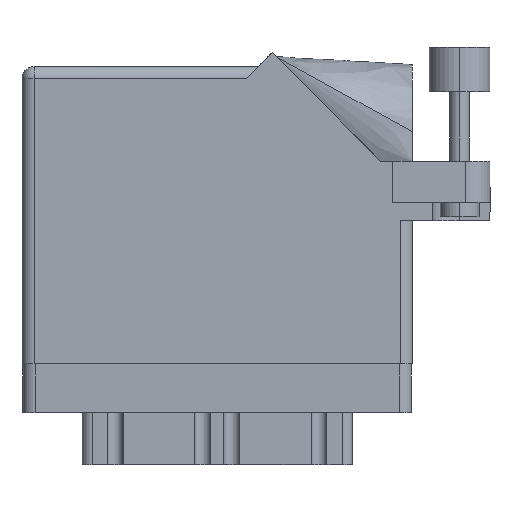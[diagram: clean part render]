
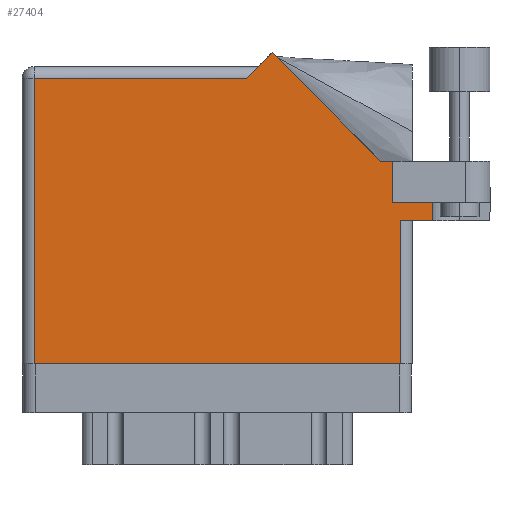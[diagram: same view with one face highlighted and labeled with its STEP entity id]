
A CAD part, front view. The second image highlights one B-rep face of the part: STEP entity #27404.
In plain terms, the highlighted face is planar.
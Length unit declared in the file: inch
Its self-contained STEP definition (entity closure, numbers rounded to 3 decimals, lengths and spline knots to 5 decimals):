
#120 = VECTOR ( 'NONE', #29337, 39.37008 ) ;
#1885 = DIRECTION ( 'NONE',  ( 1., 0., 0. ) ) ;
#2648 = VECTOR ( 'NONE', #36509, 39.37008 ) ;
#2663 = CARTESIAN_POINT ( 'NONE',  ( 1.155, 1.468, 0. ) ) ;
#3104 = CARTESIAN_POINT ( 'NONE',  ( 2.1115, 0.737, 0. ) ) ;
#4538 = VECTOR ( 'NONE', #13930, 39.37008 ) ;
#4955 = EDGE_LOOP ( 'NONE', ( #22724, #9287, #8711, #13584, #26833, #9173, #19107, #38260, #31745, #37876, #9999 ) ) ;
#5298 = EDGE_CURVE ( 'NONE', #12638, #17551, #29266, .T. ) ;
#6524 = VERTEX_POINT ( 'NONE', #27954 ) ;
#6737 = LINE ( 'NONE', #37936, #15861 ) ;
#6781 = DIRECTION ( 'NONE',  ( 0., 1., 0. ) ) ;
#7658 = CARTESIAN_POINT ( 'NONE',  ( 0., 0., 0. ) ) ;
#7851 = LINE ( 'NONE', #7658, #23454 ) ;
#8025 = CARTESIAN_POINT ( 'NONE',  ( 1.84442, 1.044, 0. ) ) ;
#8711 = ORIENTED_EDGE ( 'NONE', *, *, #5298, .T. ) ;
#9047 = CARTESIAN_POINT ( 'NONE',  ( 0.062, 0., 0. ) ) ;
#9173 = ORIENTED_EDGE ( 'NONE', *, *, #12831, .T. ) ;
#9287 = ORIENTED_EDGE ( 'NONE', *, *, #12868, .T. ) ;
#9551 = EDGE_CURVE ( 'NONE', #12047, #23862, #7851, .T. ) ;
#9591 = CARTESIAN_POINT ( 'NONE',  ( 1.84442, 1.044, 0. ) ) ;
#9999 = ORIENTED_EDGE ( 'NONE', *, *, #16222, .T. ) ;
#11290 = EDGE_CURVE ( 'NONE', #19041, #6524, #25993, .T. ) ;
#11910 = DIRECTION ( 'NONE',  ( 0., 0., -1. ) ) ;
#12047 = VERTEX_POINT ( 'NONE', #12654 ) ;
#12638 = VERTEX_POINT ( 'NONE', #26765 ) ;
#12654 = CARTESIAN_POINT ( 'NONE',  ( 0.062, 0., 0. ) ) ;
#12831 = EDGE_CURVE ( 'NONE', #19800, #26799, #34059, .T. ) ;
#12868 = EDGE_CURVE ( 'NONE', #23862, #12638, #13880, .T. ) ;
#13584 = ORIENTED_EDGE ( 'NONE', *, *, #32639, .F. ) ;
#13690 = VECTOR ( 'NONE', #35026, 39.37008 ) ;
#13880 = LINE ( 'NONE', #25952, #13690 ) ;
#13889 = DIRECTION ( 'NONE',  ( -0.707, -0.707, 0. ) ) ;
#13930 = DIRECTION ( 'NONE',  ( 1., 0., 0. ) ) ;
#14440 = EDGE_CURVE ( 'NONE', #26799, #25508, #16312, .T. ) ;
#14486 = FACE_OUTER_BOUND ( 'NONE', #4955, .T. ) ;
#14630 = CARTESIAN_POINT ( 'NONE',  ( 2.01, 0.737, 0. ) ) ;
#15861 = VECTOR ( 'NONE', #34599, 39.37008 ) ;
#16222 = EDGE_CURVE ( 'NONE', #6524, #12047, #36697, .T. ) ;
#16312 = LINE ( 'NONE', #31323, #34591 ) ;
#16725 = CARTESIAN_POINT ( 'NONE',  ( 1.91, 1.044, 0. ) ) ;
#17551 = VERTEX_POINT ( 'NONE', #3104 ) ;
#19041 = VERTEX_POINT ( 'NONE', #2663 ) ;
#19107 = ORIENTED_EDGE ( 'NONE', *, *, #14440, .T. ) ;
#19195 = EDGE_CURVE ( 'NONE', #25508, #21642, #36663, .T. ) ;
#19487 = CARTESIAN_POINT ( 'NONE',  ( 1.91, 0.831, 0. ) ) ;
#19653 = DIRECTION ( 'NONE',  ( -1., 0., 0. ) ) ;
#19800 = VERTEX_POINT ( 'NONE', #36815 ) ;
#20468 = CARTESIAN_POINT ( 'NONE',  ( 1.28771, 1.60071, 0. ) ) ;
#20619 = CARTESIAN_POINT ( 'NONE',  ( 0., 1.53, 0. ) ) ;
#21258 = VECTOR ( 'NONE', #6781, 39.37008 ) ;
#21642 = VERTEX_POINT ( 'NONE', #20468 ) ;
#22028 = LINE ( 'NONE', #28537, #38884 ) ;
#22724 = ORIENTED_EDGE ( 'NONE', *, *, #9551, .T. ) ;
#23454 = VECTOR ( 'NONE', #1885, 39.37008 ) ;
#23818 = AXIS2_PLACEMENT_3D ( 'NONE', #20619, #11910, #36594 ) ;
#23862 = VERTEX_POINT ( 'NONE', #35208 ) ;
#25508 = VERTEX_POINT ( 'NONE', #8025 ) ;
#25828 = LINE ( 'NONE', #19487, #4538 ) ;
#25909 = EDGE_CURVE ( 'NONE', #21642, #19041, #22028, .T. ) ;
#25952 = CARTESIAN_POINT ( 'NONE',  ( 1.948, 0.737, 0. ) ) ;
#25993 = LINE ( 'NONE', #29141, #120 ) ;
#26304 = DIRECTION ( 'NONE',  ( 1., 0., 0. ) ) ;
#26765 = CARTESIAN_POINT ( 'NONE',  ( 1.948, 0.737, 0. ) ) ;
#26799 = VERTEX_POINT ( 'NONE', #16725 ) ;
#26833 = ORIENTED_EDGE ( 'NONE', *, *, #33588, .F. ) ;
#27404 = ADVANCED_FACE ( 'NONE', ( #14486 ), #38576, .F. ) ;
#27954 = CARTESIAN_POINT ( 'NONE',  ( 0.062, 1.468, 0. ) ) ;
#28171 = VECTOR ( 'NONE', #26304, 39.37008 ) ;
#28537 = CARTESIAN_POINT ( 'NONE',  ( 1.217, 1.53, 0. ) ) ;
#29141 = CARTESIAN_POINT ( 'NONE',  ( 0., 1.468, 0. ) ) ;
#29266 = LINE ( 'NONE', #14630, #28171 ) ;
#29337 = DIRECTION ( 'NONE',  ( -1., 0., 0. ) ) ;
#31323 = CARTESIAN_POINT ( 'NONE',  ( 2.41, 1.044, 0. ) ) ;
#31745 = ORIENTED_EDGE ( 'NONE', *, *, #25909, .T. ) ;
#32639 = EDGE_CURVE ( 'NONE', #35351, #17551, #6737, .T. ) ;
#32737 = VECTOR ( 'NONE', #36863, 39.37008 ) ;
#33574 = CARTESIAN_POINT ( 'NONE',  ( 2.1115, 0.831, 0. ) ) ;
#33588 = EDGE_CURVE ( 'NONE', #19800, #35351, #25828, .T. ) ;
#33860 = CARTESIAN_POINT ( 'NONE',  ( 1.91, 0.831, 0. ) ) ;
#34059 = LINE ( 'NONE', #33860, #21258 ) ;
#34591 = VECTOR ( 'NONE', #19653, 39.37008 ) ;
#34599 = DIRECTION ( 'NONE',  ( 0., -1., 0. ) ) ;
#35026 = DIRECTION ( 'NONE',  ( 0., 1., 0. ) ) ;
#35208 = CARTESIAN_POINT ( 'NONE',  ( 1.948, 0., 0. ) ) ;
#35351 = VERTEX_POINT ( 'NONE', #33574 ) ;
#36509 = DIRECTION ( 'NONE',  ( 0., -1., 0. ) ) ;
#36594 = DIRECTION ( 'NONE',  ( -1., 0., 0. ) ) ;
#36663 = LINE ( 'NONE', #9591, #32737 ) ;
#36697 = LINE ( 'NONE', #9047, #2648 ) ;
#36815 = CARTESIAN_POINT ( 'NONE',  ( 1.91, 0.831, 0. ) ) ;
#36863 = DIRECTION ( 'NONE',  ( -0.707, 0.707, 0. ) ) ;
#37876 = ORIENTED_EDGE ( 'NONE', *, *, #11290, .T. ) ;
#37936 = CARTESIAN_POINT ( 'NONE',  ( 2.1115, 1.16177, 0. ) ) ;
#38260 = ORIENTED_EDGE ( 'NONE', *, *, #19195, .T. ) ;
#38576 = PLANE ( 'NONE',  #23818 ) ;
#38884 = VECTOR ( 'NONE', #13889, 39.37008 ) ;
